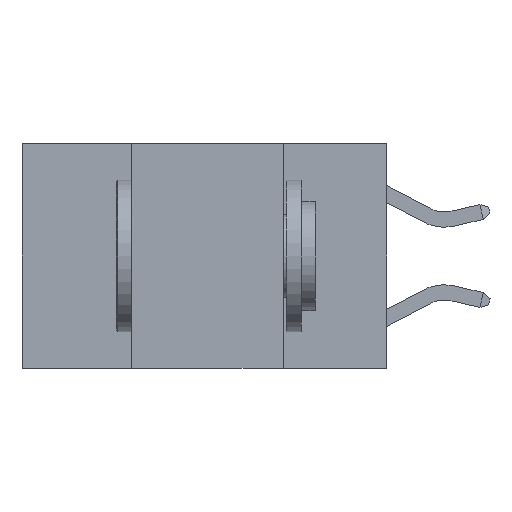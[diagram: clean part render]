
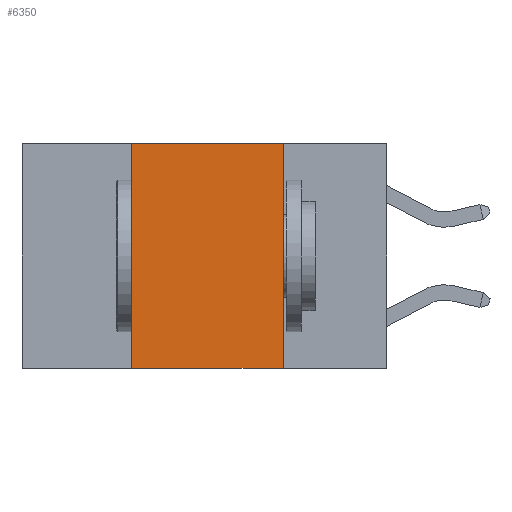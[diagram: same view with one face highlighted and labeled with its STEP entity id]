
A CAD part, left-side view. The second image highlights one B-rep face of the part: STEP entity #6350.
In plain terms, the highlighted planar face has unit normal (-1, 0, 0).
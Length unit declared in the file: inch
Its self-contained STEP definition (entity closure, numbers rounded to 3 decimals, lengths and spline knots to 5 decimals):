
#86 = LINE ( 'NONE', #6099, #2242 ) ;
#721 = LINE ( 'NONE', #7394, #5217 ) ;
#1995 = ORIENTED_EDGE ( 'NONE', *, *, #7512, .F. ) ;
#2242 = VECTOR ( 'NONE', #10550, 39.37008 ) ;
#2312 = AXIS2_PLACEMENT_3D ( 'NONE', #3797, #10911, #5623 ) ;
#2425 = VECTOR ( 'NONE', #5249, 39.37008 ) ;
#2553 = CARTESIAN_POINT ( 'NONE',  ( 0., 0.6, -0.37 ) ) ;
#2627 = VERTEX_POINT ( 'NONE', #9995 ) ;
#2630 = CARTESIAN_POINT ( 'NONE',  ( 0., 0.6, 0. ) ) ;
#2902 = PLANE ( 'NONE',  #2312 ) ;
#2925 = VERTEX_POINT ( 'NONE', #7463 ) ;
#3797 = CARTESIAN_POINT ( 'NONE',  ( 0., 0.6, 0. ) ) ;
#4091 = FACE_OUTER_BOUND ( 'NONE', #11069, .T. ) ;
#4202 = VECTOR ( 'NONE', #8944, 39.37008 ) ;
#4232 = LINE ( 'NONE', #2553, #2425 ) ;
#4461 = CARTESIAN_POINT ( 'NONE',  ( 0., 0.42, -0.37 ) ) ;
#5015 = EDGE_CURVE ( 'NONE', #7522, #2627, #721, .T. ) ;
#5217 = VECTOR ( 'NONE', #8273, 39.37008 ) ;
#5249 = DIRECTION ( 'NONE',  ( 0., -1., 0. ) ) ;
#5623 = DIRECTION ( 'NONE',  ( 0., 0., -1. ) ) ;
#6078 = EDGE_CURVE ( 'NONE', #7522, #2925, #4232, .T. ) ;
#6099 = CARTESIAN_POINT ( 'NONE',  ( 0., 0.17, 0. ) ) ;
#6350 = ADVANCED_FACE ( 'NONE', ( #4091 ), #2902, .F. ) ;
#6503 = ORIENTED_EDGE ( 'NONE', *, *, #9235, .F. ) ;
#6789 = ORIENTED_EDGE ( 'NONE', *, *, #5015, .F. ) ;
#7394 = CARTESIAN_POINT ( 'NONE',  ( 0., 0.42, 0. ) ) ;
#7463 = CARTESIAN_POINT ( 'NONE',  ( 0., 0.17, -0.37 ) ) ;
#7512 = EDGE_CURVE ( 'NONE', #2627, #8636, #10740, .T. ) ;
#7522 = VERTEX_POINT ( 'NONE', #4461 ) ;
#8273 = DIRECTION ( 'NONE',  ( 0., 0., 1. ) ) ;
#8636 = VERTEX_POINT ( 'NONE', #9723 ) ;
#8944 = DIRECTION ( 'NONE',  ( 0., -1., 0. ) ) ;
#9149 = ORIENTED_EDGE ( 'NONE', *, *, #6078, .T. ) ;
#9235 = EDGE_CURVE ( 'NONE', #8636, #2925, #86, .T. ) ;
#9723 = CARTESIAN_POINT ( 'NONE',  ( 0., 0.17, 0. ) ) ;
#9995 = CARTESIAN_POINT ( 'NONE',  ( 0., 0.42, 0. ) ) ;
#10550 = DIRECTION ( 'NONE',  ( 0., 0., -1. ) ) ;
#10740 = LINE ( 'NONE', #2630, #4202 ) ;
#10911 = DIRECTION ( 'NONE',  ( 1., 0., 0. ) ) ;
#11069 = EDGE_LOOP ( 'NONE', ( #6503, #1995, #6789, #9149 ) ) ;
